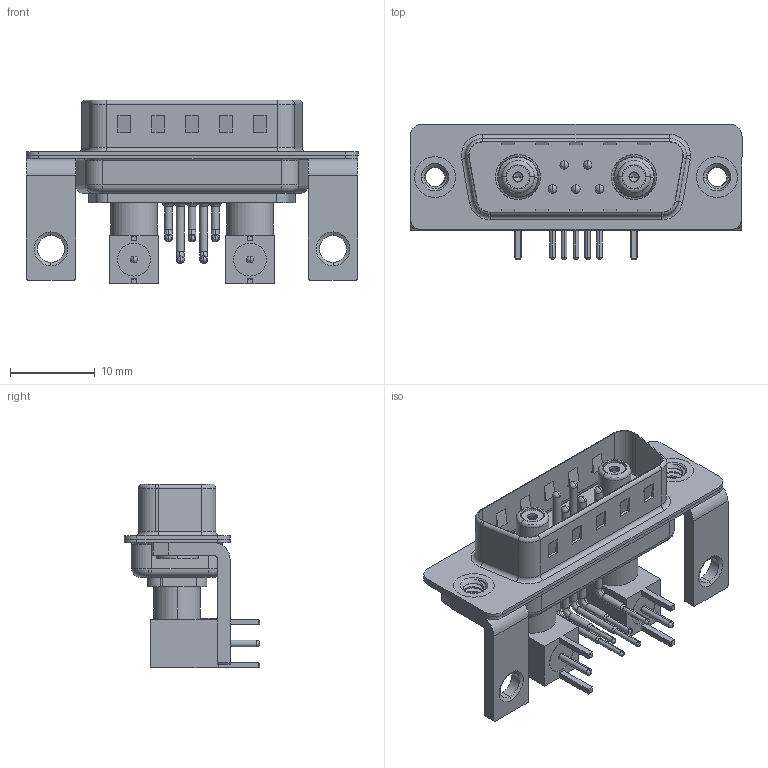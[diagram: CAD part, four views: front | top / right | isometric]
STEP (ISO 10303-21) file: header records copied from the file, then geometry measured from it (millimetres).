
FILE_DESCRIPTION (( 'STEP AP203' ), '1' );
FILE_NAME ('629-7W2-640-5N4.STEP', '2022-05-06T17:28:30', ( '' ), ( '' ), 'SwSTEP 2.0', 'SolidWorks 2020', '' );
FILE_SCHEMA (( 'CONFIG_CONTROL_DESIGN' ));
Length unit declared in the file: millimetre
Products named in the file (17): 629Combo Contact Row 1; Insulator Socket; Co-Ax Jack_RA PC Tail; RA Back Shell; 629Combo Threaded Rivet_3; 629Combo Stabilizer Bracket; 629Combo Contact Row 2; Socket_RA; 629Combo Shell Rear_15 Contacts; Co-Ax Jack Assy_RA; 629Combo Shell Front_15 Contacts; Insulator RA Pin; 629-7W2-640-5N4; 629Combo Housing_7W2; Insulator Socket 2; Locking Collar
Assembly tree (28 placements, depth 3):
  629-7W2-640-5N4
    629Combo Housing_7W2
    629Combo Shell Rear_15 Contacts
    629Combo Shell Front_15 Contacts
    629Combo Threaded Rivet_3  x2
    629Combo Stabilizer Bracket  x2
    Co-Ax Jack Assy_RA
      Co-Ax Jack_RA PC Tail
      Insulator Socket
      Insulator Socket 2
      Locking Collar
      Socket_RA
      RA Back Shell
      Insulator RA Pin
    Co-Ax Jack Assy_RA
      Co-Ax Jack_RA PC Tail
      Insulator Socket
      Insulator Socket 2
      Locking Collar
      Socket_RA
      RA Back Shell
      Insulator RA Pin
    629Combo Contact Row 1  x2
    629Combo Contact Row 2  x3
Bounding box: 39.2 x 16 x 21.71 mm (x, y, z)
Volume: 2718.4 mm3; surface area: 7369.7 mm2
Topology: 26 solids, 26 shells, 1234 faces, 3207 edges, 2048 vertices
Faces by surface type: plane 593, cylinder 465, cone 72, torus 62, bspline 38, sphere 4
Entity records: 25897 total; most frequent: CARTESIAN_POINT 5625, DIRECTION 3958, ORIENTED_EDGE 3684, EDGE_CURVE 1842, AXIS2_PLACEMENT_3D 1430, VERTEX_POINT 1182, LINE 1098, VECTOR 1098
